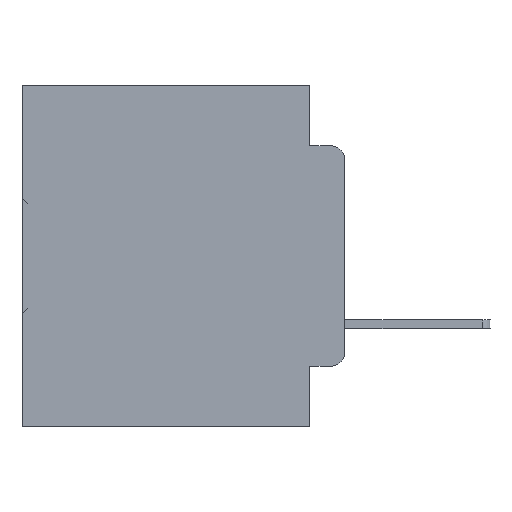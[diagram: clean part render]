
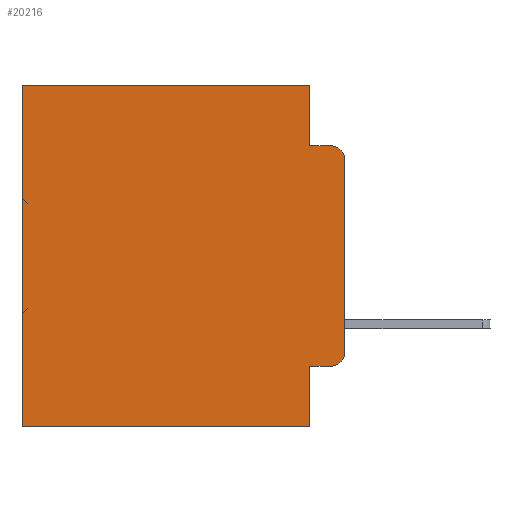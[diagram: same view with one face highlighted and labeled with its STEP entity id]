
A CAD part, left-side view. The second image highlights one B-rep face of the part: STEP entity #20216.
In plain terms, the highlighted planar face has unit normal (-1, 0, 0).
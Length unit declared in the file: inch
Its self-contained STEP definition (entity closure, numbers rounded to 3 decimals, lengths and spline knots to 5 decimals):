
#373 = EDGE_CURVE ( 'NONE', #29855, #29677, #35283, .T. ) ;
#1449 = CARTESIAN_POINT ( 'NONE',  ( 0.298, 0., -0.5 ) ) ;
#1976 = ORIENTED_EDGE ( 'NONE', *, *, #35685, .T. ) ;
#2192 = LINE ( 'NONE', #29816, #30296 ) ;
#2326 = VERTEX_POINT ( 'NONE', #34698 ) ;
#2434 = ORIENTED_EDGE ( 'NONE', *, *, #13720, .T. ) ;
#3313 = VECTOR ( 'NONE', #24067, 39.37008 ) ;
#3517 = DIRECTION ( 'NONE',  ( 0., -1., 0. ) ) ;
#3864 = VECTOR ( 'NONE', #21347, 39.37008 ) ;
#4183 = ORIENTED_EDGE ( 'NONE', *, *, #12344, .F. ) ;
#4224 = DIRECTION ( 'NONE',  ( 0., 1., 0. ) ) ;
#5108 = VERTEX_POINT ( 'NONE', #15689 ) ;
#5467 = VERTEX_POINT ( 'NONE', #23034 ) ;
#6557 = CARTESIAN_POINT ( 'NONE',  ( 0.298, 0.02, -0.3915 ) ) ;
#7196 = ORIENTED_EDGE ( 'NONE', *, *, #33873, .F. ) ;
#8078 = CARTESIAN_POINT ( 'NONE',  ( 0.298, 0.051, 0. ) ) ;
#8229 = PLANE ( 'NONE',  #15519 ) ;
#8948 = ORIENTED_EDGE ( 'NONE', *, *, #373, .T. ) ;
#9383 = DIRECTION ( 'NONE',  ( 0., 0., -1. ) ) ;
#9628 = CARTESIAN_POINT ( 'NONE',  ( 0.298, 0.473, 0. ) ) ;
#9635 = VECTOR ( 'NONE', #3517, 39.37008 ) ;
#10517 = CARTESIAN_POINT ( 'NONE',  ( 0.298, 0.02, -0.0885 ) ) ;
#10952 = DIRECTION ( 'NONE',  ( 0., 0., -1. ) ) ;
#11096 = DIRECTION ( 'NONE',  ( 1., 0., 0. ) ) ;
#11849 = EDGE_CURVE ( 'NONE', #33617, #14032, #32050, .T. ) ;
#12344 = EDGE_CURVE ( 'NONE', #5467, #30380, #14443, .T. ) ;
#12441 = CARTESIAN_POINT ( 'NONE',  ( 0.298, 0.02, -0.1085 ) ) ;
#13004 = VECTOR ( 'NONE', #22369, 39.37008 ) ;
#13160 = VERTEX_POINT ( 'NONE', #10517 ) ;
#13214 = CIRCLE ( 'NONE', #26704, 0.02 ) ;
#13312 = CARTESIAN_POINT ( 'NONE',  ( 0.298, 0.051, 0. ) ) ;
#13720 = EDGE_CURVE ( 'NONE', #29677, #30380, #18842, .T. ) ;
#14032 = VERTEX_POINT ( 'NONE', #34088 ) ;
#14264 = ORIENTED_EDGE ( 'NONE', *, *, #31365, .T. ) ;
#14443 = LINE ( 'NONE', #1449, #28559 ) ;
#14638 = VECTOR ( 'NONE', #29461, 39.37008 ) ;
#15293 = DIRECTION ( 'NONE',  ( 0., 0., -1. ) ) ;
#15351 = CIRCLE ( 'NONE', #33497, 0.02 ) ;
#15519 = AXIS2_PLACEMENT_3D ( 'NONE', #27970, #11096, #30754 ) ;
#15689 = CARTESIAN_POINT ( 'NONE',  ( 0.298, 0.051, -0.0885 ) ) ;
#16044 = ORIENTED_EDGE ( 'NONE', *, *, #16362, .F. ) ;
#16362 = EDGE_CURVE ( 'NONE', #26797, #2326, #27858, .T. ) ;
#16848 = CARTESIAN_POINT ( 'NONE',  ( 0.298, 0., -0.1085 ) ) ;
#17395 = ORIENTED_EDGE ( 'NONE', *, *, #33181, .F. ) ;
#18277 = CARTESIAN_POINT ( 'NONE',  ( 0.298, 0.051, -0.4115 ) ) ;
#18842 = LINE ( 'NONE', #29919, #3864 ) ;
#19150 = ORIENTED_EDGE ( 'NONE', *, *, #11849, .T. ) ;
#19154 = LINE ( 'NONE', #35189, #3313 ) ;
#20216 = ADVANCED_FACE ( 'NONE', ( #31615 ), #8229, .F. ) ;
#20357 = EDGE_LOOP ( 'NONE', ( #16044, #1976, #33506, #7196, #8948, #2434, #4183, #17395, #19150, #14264 ) ) ;
#21297 = CARTESIAN_POINT ( 'NONE',  ( 0.298, 0.473, -0.5 ) ) ;
#21347 = DIRECTION ( 'NONE',  ( 0., 0., -1. ) ) ;
#22369 = DIRECTION ( 'NONE',  ( 0., 1., 0. ) ) ;
#23034 = CARTESIAN_POINT ( 'NONE',  ( 0.298, 0.051, -0.5 ) ) ;
#24067 = DIRECTION ( 'NONE',  ( 0., 0., -1. ) ) ;
#25057 = EDGE_CURVE ( 'NONE', #5108, #13160, #2192, .T. ) ;
#26141 = LINE ( 'NONE', #8078, #32623 ) ;
#26288 = DIRECTION ( 'NONE',  ( -1., 0., 0. ) ) ;
#26649 = CARTESIAN_POINT ( 'NONE',  ( 0.298, 0., 0. ) ) ;
#26704 = AXIS2_PLACEMENT_3D ( 'NONE', #12441, #32059, #15293 ) ;
#26797 = VERTEX_POINT ( 'NONE', #16848 ) ;
#27858 = LINE ( 'NONE', #26649, #14638 ) ;
#27970 = CARTESIAN_POINT ( 'NONE',  ( 0.298, 0., 0. ) ) ;
#28559 = VECTOR ( 'NONE', #4224, 39.37008 ) ;
#29461 = DIRECTION ( 'NONE',  ( 0., 0., -1. ) ) ;
#29677 = VERTEX_POINT ( 'NONE', #9628 ) ;
#29816 = CARTESIAN_POINT ( 'NONE',  ( 0.298, 0.051, -0.0885 ) ) ;
#29855 = VERTEX_POINT ( 'NONE', #13312 ) ;
#29919 = CARTESIAN_POINT ( 'NONE',  ( 0.298, 0.473, 0. ) ) ;
#29927 = DIRECTION ( 'NONE',  ( 0., -1., 0. ) ) ;
#30296 = VECTOR ( 'NONE', #29927, 39.37008 ) ;
#30380 = VERTEX_POINT ( 'NONE', #21297 ) ;
#30754 = DIRECTION ( 'NONE',  ( 0., 0., -1. ) ) ;
#31200 = CARTESIAN_POINT ( 'NONE',  ( 0.298, 0., 0. ) ) ;
#31365 = EDGE_CURVE ( 'NONE', #14032, #2326, #15351, .T. ) ;
#31615 = FACE_OUTER_BOUND ( 'NONE', #20357, .T. ) ;
#32050 = LINE ( 'NONE', #34228, #9635 ) ;
#32059 = DIRECTION ( 'NONE',  ( -1., 0., 0. ) ) ;
#32623 = VECTOR ( 'NONE', #10952, 39.37008 ) ;
#33181 = EDGE_CURVE ( 'NONE', #33617, #5467, #19154, .T. ) ;
#33497 = AXIS2_PLACEMENT_3D ( 'NONE', #6557, #26288, #9383 ) ;
#33506 = ORIENTED_EDGE ( 'NONE', *, *, #25057, .F. ) ;
#33617 = VERTEX_POINT ( 'NONE', #18277 ) ;
#33873 = EDGE_CURVE ( 'NONE', #29855, #5108, #26141, .T. ) ;
#34088 = CARTESIAN_POINT ( 'NONE',  ( 0.298, 0.02, -0.4115 ) ) ;
#34228 = CARTESIAN_POINT ( 'NONE',  ( 0.298, 0.051, -0.4115 ) ) ;
#34698 = CARTESIAN_POINT ( 'NONE',  ( 0.298, 0., -0.3915 ) ) ;
#35189 = CARTESIAN_POINT ( 'NONE',  ( 0.298, 0.051, 0. ) ) ;
#35283 = LINE ( 'NONE', #31200, #13004 ) ;
#35685 = EDGE_CURVE ( 'NONE', #26797, #13160, #13214, .T. ) ;
